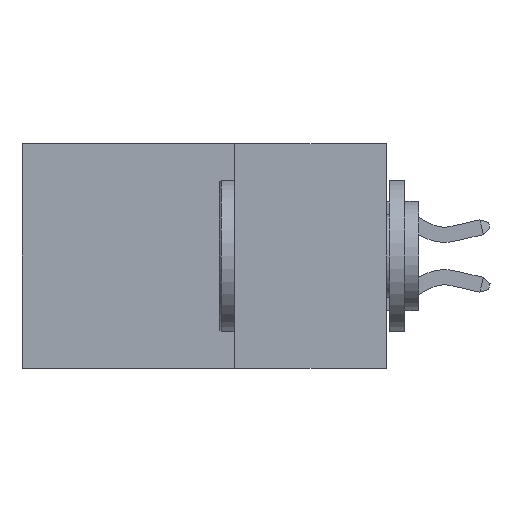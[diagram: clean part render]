
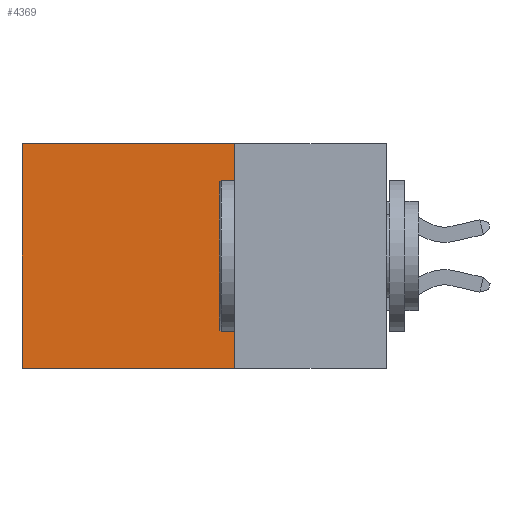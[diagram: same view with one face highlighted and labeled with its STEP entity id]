
A CAD part, left-side view. The second image highlights one B-rep face of the part: STEP entity #4369.
In plain terms, the highlighted planar face has unit normal (-1, 0, 0).
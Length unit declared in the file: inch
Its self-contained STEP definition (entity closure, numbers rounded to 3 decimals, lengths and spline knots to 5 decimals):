
#617 = DIRECTION ( 'NONE',  ( 0., 0., -1. ) ) ;
#2644 = PLANE ( 'NONE',  #20216 ) ;
#4164 = CARTESIAN_POINT ( 'NONE',  ( 0.298, 0.25, 0. ) ) ;
#4369 = ADVANCED_FACE ( 'NONE', ( #6648 ), #2644, .F. ) ;
#4783 = CARTESIAN_POINT ( 'NONE',  ( 0.298, 0.6, 0. ) ) ;
#4876 = VERTEX_POINT ( 'NONE', #15972 ) ;
#5495 = EDGE_LOOP ( 'NONE', ( #23751, #11894, #11974, #20254 ) ) ;
#5523 = LINE ( 'NONE', #7432, #5795 ) ;
#5725 = VERTEX_POINT ( 'NONE', #14283 ) ;
#5795 = VECTOR ( 'NONE', #13367, 39.37008 ) ;
#6648 = FACE_OUTER_BOUND ( 'NONE', #5495, .T. ) ;
#7432 = CARTESIAN_POINT ( 'NONE',  ( 0.298, 0.25, 0. ) ) ;
#8385 = CARTESIAN_POINT ( 'NONE',  ( 0.298, 0.25, 0. ) ) ;
#9156 = LINE ( 'NONE', #23974, #19471 ) ;
#9670 = LINE ( 'NONE', #23058, #19935 ) ;
#11487 = DIRECTION ( 'NONE',  ( 0., 1., 0. ) ) ;
#11610 = EDGE_CURVE ( 'NONE', #4876, #23575, #5523, .T. ) ;
#11792 = VECTOR ( 'NONE', #13881, 39.37008 ) ;
#11894 = ORIENTED_EDGE ( 'NONE', *, *, #21848, .F. ) ;
#11974 = ORIENTED_EDGE ( 'NONE', *, *, #11610, .F. ) ;
#13045 = EDGE_CURVE ( 'NONE', #4876, #18930, #14818, .T. ) ;
#13367 = DIRECTION ( 'NONE',  ( 0., 0., -1. ) ) ;
#13881 = DIRECTION ( 'NONE',  ( 0., 1., 0. ) ) ;
#14283 = CARTESIAN_POINT ( 'NONE',  ( 0.298, 0.6, -0.37 ) ) ;
#14358 = DIRECTION ( 'NONE',  ( 0., 0., -1. ) ) ;
#14703 = CARTESIAN_POINT ( 'NONE',  ( 0.298, 0.25, -0.37 ) ) ;
#14818 = LINE ( 'NONE', #4164, #11792 ) ;
#15972 = CARTESIAN_POINT ( 'NONE',  ( 0.298, 0.25, 0. ) ) ;
#18152 = DIRECTION ( 'NONE',  ( 1., 0., 0. ) ) ;
#18928 = EDGE_CURVE ( 'NONE', #18930, #5725, #9156, .T. ) ;
#18930 = VERTEX_POINT ( 'NONE', #4783 ) ;
#19471 = VECTOR ( 'NONE', #617, 39.37008 ) ;
#19935 = VECTOR ( 'NONE', #11487, 39.37008 ) ;
#20216 = AXIS2_PLACEMENT_3D ( 'NONE', #8385, #18152, #14358 ) ;
#20254 = ORIENTED_EDGE ( 'NONE', *, *, #13045, .T. ) ;
#21848 = EDGE_CURVE ( 'NONE', #23575, #5725, #9670, .T. ) ;
#23058 = CARTESIAN_POINT ( 'NONE',  ( 0.298, 0.25, -0.37 ) ) ;
#23575 = VERTEX_POINT ( 'NONE', #14703 ) ;
#23751 = ORIENTED_EDGE ( 'NONE', *, *, #18928, .T. ) ;
#23974 = CARTESIAN_POINT ( 'NONE',  ( 0.298, 0.6, 0. ) ) ;
